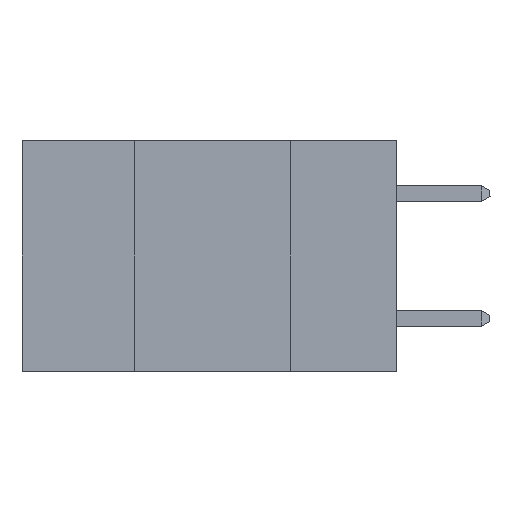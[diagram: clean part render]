
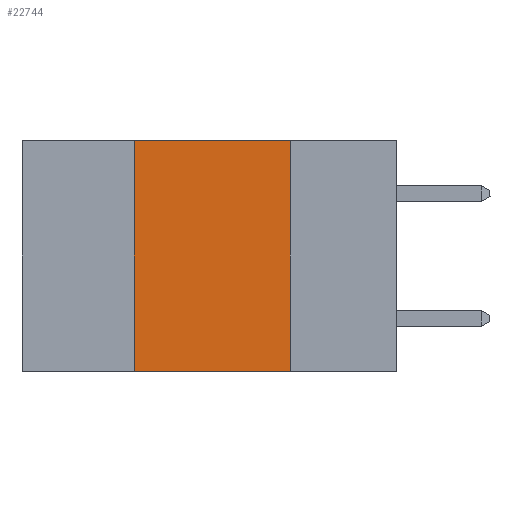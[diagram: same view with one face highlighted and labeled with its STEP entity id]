
A CAD part, left-side view. The second image highlights one B-rep face of the part: STEP entity #22744.
In plain terms, the highlighted planar face has unit normal (-1, 0, 0).
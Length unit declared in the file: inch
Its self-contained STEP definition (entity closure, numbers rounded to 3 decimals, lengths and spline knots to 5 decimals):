
#655 = LINE ( 'NONE', #19808, #8373 ) ;
#862 = CARTESIAN_POINT ( 'NONE',  ( 0., 0.6, -0.37 ) ) ;
#3028 = CARTESIAN_POINT ( 'NONE',  ( 0., 0.17, 0. ) ) ;
#5206 = EDGE_LOOP ( 'NONE', ( #11750, #12429, #23692, #8129 ) ) ;
#5400 = VERTEX_POINT ( 'NONE', #6247 ) ;
#5535 = VECTOR ( 'NONE', #23236, 39.37008 ) ;
#5575 = CARTESIAN_POINT ( 'NONE',  ( 0., 0.6, 0. ) ) ;
#5911 = CARTESIAN_POINT ( 'NONE',  ( 0., 0.42, -0.37 ) ) ;
#6247 = CARTESIAN_POINT ( 'NONE',  ( 0., 0.42, 0. ) ) ;
#6301 = CARTESIAN_POINT ( 'NONE',  ( 0., 0.6, 0. ) ) ;
#7708 = DIRECTION ( 'NONE',  ( 0., 0., -1. ) ) ;
#8129 = ORIENTED_EDGE ( 'NONE', *, *, #26190, .T. ) ;
#8373 = VECTOR ( 'NONE', #26130, 39.37008 ) ;
#10632 = VERTEX_POINT ( 'NONE', #5911 ) ;
#11593 = VERTEX_POINT ( 'NONE', #19218 ) ;
#11750 = ORIENTED_EDGE ( 'NONE', *, *, #23386, .F. ) ;
#12429 = ORIENTED_EDGE ( 'NONE', *, *, #21619, .F. ) ;
#13084 = VECTOR ( 'NONE', #24149, 39.37008 ) ;
#13764 = LINE ( 'NONE', #862, #13084 ) ;
#14097 = LINE ( 'NONE', #3028, #23977 ) ;
#14553 = VERTEX_POINT ( 'NONE', #20896 ) ;
#16208 = PLANE ( 'NONE',  #17682 ) ;
#16885 = LINE ( 'NONE', #6301, #5535 ) ;
#17682 = AXIS2_PLACEMENT_3D ( 'NONE', #5575, #20436, #7708 ) ;
#18801 = FACE_OUTER_BOUND ( 'NONE', #5206, .T. ) ;
#19218 = CARTESIAN_POINT ( 'NONE',  ( 0., 0.17, -0.37 ) ) ;
#19808 = CARTESIAN_POINT ( 'NONE',  ( 0., 0.42, 0. ) ) ;
#20117 = DIRECTION ( 'NONE',  ( 0., 0., -1. ) ) ;
#20436 = DIRECTION ( 'NONE',  ( 1., 0., 0. ) ) ;
#20896 = CARTESIAN_POINT ( 'NONE',  ( 0., 0.17, 0. ) ) ;
#21619 = EDGE_CURVE ( 'NONE', #5400, #14553, #16885, .T. ) ;
#22744 = ADVANCED_FACE ( 'NONE', ( #18801 ), #16208, .F. ) ;
#23236 = DIRECTION ( 'NONE',  ( 0., -1., 0. ) ) ;
#23386 = EDGE_CURVE ( 'NONE', #14553, #11593, #14097, .T. ) ;
#23692 = ORIENTED_EDGE ( 'NONE', *, *, #24795, .F. ) ;
#23977 = VECTOR ( 'NONE', #20117, 39.37008 ) ;
#24149 = DIRECTION ( 'NONE',  ( 0., -1., 0. ) ) ;
#24795 = EDGE_CURVE ( 'NONE', #10632, #5400, #655, .T. ) ;
#26130 = DIRECTION ( 'NONE',  ( 0., 0., 1. ) ) ;
#26190 = EDGE_CURVE ( 'NONE', #10632, #11593, #13764, .T. ) ;
